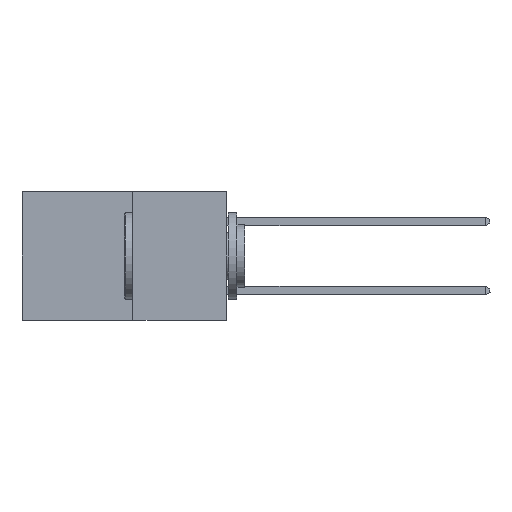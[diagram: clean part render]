
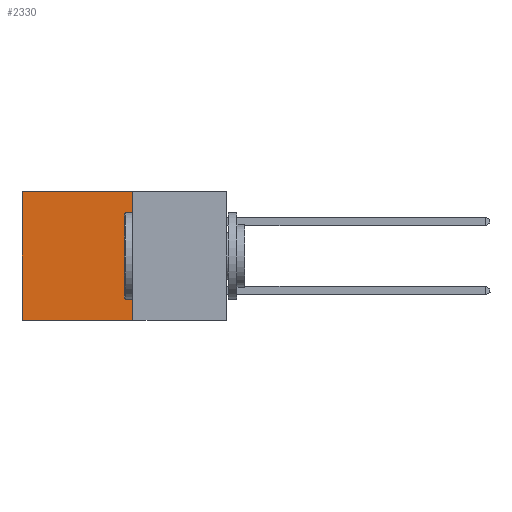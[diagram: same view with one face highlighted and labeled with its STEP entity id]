
A CAD part, left-side view. The second image highlights one B-rep face of the part: STEP entity #2330.
In plain terms, the highlighted planar face has unit normal (-1, 0, 0).
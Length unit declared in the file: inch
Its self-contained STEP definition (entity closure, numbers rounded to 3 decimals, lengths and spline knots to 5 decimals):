
#317 = VECTOR ( 'NONE', #1656, 39.37008 ) ;
#825 = CARTESIAN_POINT ( 'NONE',  ( 0.277, 0.59, -0.37 ) ) ;
#1396 = ORIENTED_EDGE ( 'NONE', *, *, #8201, .T. ) ;
#1652 = LINE ( 'NONE', #8602, #7875 ) ;
#1656 = DIRECTION ( 'NONE',  ( 0., 0., -1. ) ) ;
#1901 = VERTEX_POINT ( 'NONE', #9127 ) ;
#2076 = AXIS2_PLACEMENT_3D ( 'NONE', #9626, #9119, #9105 ) ;
#2330 = ADVANCED_FACE ( 'NONE', ( #9814 ), #9208, .F. ) ;
#2843 = VECTOR ( 'NONE', #6119, 39.37008 ) ;
#3548 = ORIENTED_EDGE ( 'NONE', *, *, #4085, .F. ) ;
#3795 = CARTESIAN_POINT ( 'NONE',  ( 0.277, 0.27, -0.37 ) ) ;
#4024 = CARTESIAN_POINT ( 'NONE',  ( 0.277, 0.27, 0. ) ) ;
#4085 = EDGE_CURVE ( 'NONE', #5998, #1901, #9236, .T. ) ;
#4119 = CARTESIAN_POINT ( 'NONE',  ( 0.277, 0.27, -0.37 ) ) ;
#4245 = DIRECTION ( 'NONE',  ( 0., 0., -1. ) ) ;
#4327 = EDGE_CURVE ( 'NONE', #8172, #4524, #9645, .T. ) ;
#4524 = VERTEX_POINT ( 'NONE', #9584 ) ;
#4566 = EDGE_CURVE ( 'NONE', #8172, #5998, #1652, .T. ) ;
#4768 = LINE ( 'NONE', #825, #317 ) ;
#5295 = VECTOR ( 'NONE', #7165, 39.37008 ) ;
#5678 = EDGE_LOOP ( 'NONE', ( #1396, #3548, #7872, #9831 ) ) ;
#5998 = VERTEX_POINT ( 'NONE', #3795 ) ;
#6119 = DIRECTION ( 'NONE',  ( 0., 1., 0. ) ) ;
#7165 = DIRECTION ( 'NONE',  ( 0., 1., 0. ) ) ;
#7872 = ORIENTED_EDGE ( 'NONE', *, *, #4566, .F. ) ;
#7875 = VECTOR ( 'NONE', #4245, 39.37008 ) ;
#8172 = VERTEX_POINT ( 'NONE', #4024 ) ;
#8201 = EDGE_CURVE ( 'NONE', #4524, #1901, #4768, .T. ) ;
#8602 = CARTESIAN_POINT ( 'NONE',  ( 0.277, 0.27, -0.37 ) ) ;
#8818 = CARTESIAN_POINT ( 'NONE',  ( 0.277, 0.27, 0. ) ) ;
#9105 = DIRECTION ( 'NONE',  ( 0., 0., -1. ) ) ;
#9119 = DIRECTION ( 'NONE',  ( 1., 0., 0. ) ) ;
#9127 = CARTESIAN_POINT ( 'NONE',  ( 0.277, 0.59, -0.37 ) ) ;
#9208 = PLANE ( 'NONE',  #2076 ) ;
#9236 = LINE ( 'NONE', #4119, #2843 ) ;
#9584 = CARTESIAN_POINT ( 'NONE',  ( 0.277, 0.59, 0. ) ) ;
#9626 = CARTESIAN_POINT ( 'NONE',  ( 0.277, 0.27, -0.37 ) ) ;
#9645 = LINE ( 'NONE', #8818, #5295 ) ;
#9814 = FACE_OUTER_BOUND ( 'NONE', #5678, .T. ) ;
#9831 = ORIENTED_EDGE ( 'NONE', *, *, #4327, .T. ) ;
